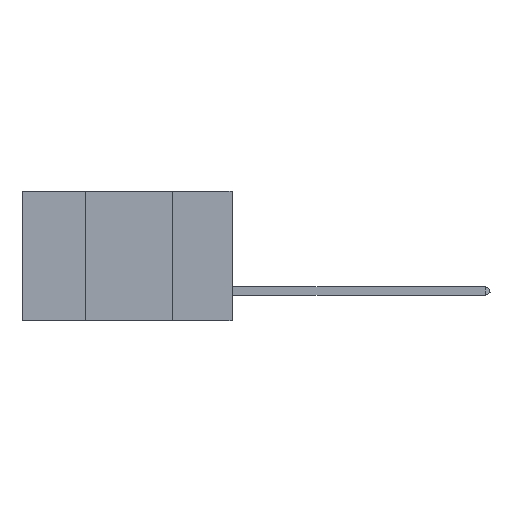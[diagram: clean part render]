
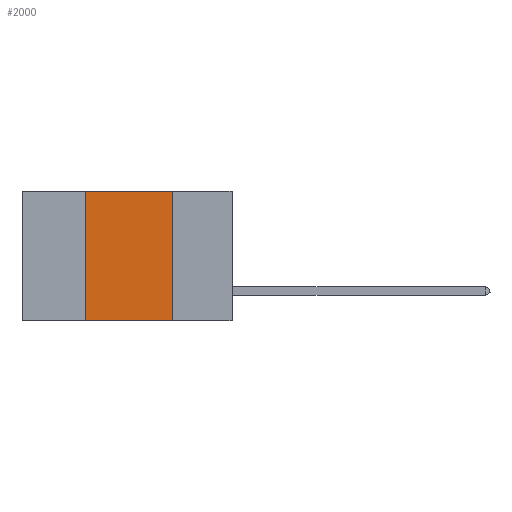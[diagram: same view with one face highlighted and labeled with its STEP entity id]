
A CAD part, left-side view. The second image highlights one B-rep face of the part: STEP entity #2000.
In plain terms, the highlighted planar face has unit normal (-1, 0, 0).
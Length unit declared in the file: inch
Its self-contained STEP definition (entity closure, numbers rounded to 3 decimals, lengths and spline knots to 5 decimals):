
#184 = PLANE ( 'NONE',  #1327 ) ;
#1327 = AXIS2_PLACEMENT_3D ( 'NONE', #18711, #16907, #7871 ) ;
#1763 = VERTEX_POINT ( 'NONE', #6964 ) ;
#2000 = ADVANCED_FACE ( 'NONE', ( #18683 ), #184, .F. ) ;
#2273 = VECTOR ( 'NONE', #9489, 39.37008 ) ;
#4126 = EDGE_CURVE ( 'NONE', #18324, #16818, #17830, .T. ) ;
#4892 = CARTESIAN_POINT ( 'NONE',  ( 0., 0.6, -0.37 ) ) ;
#5587 = CARTESIAN_POINT ( 'NONE',  ( 0., 0.17, 0. ) ) ;
#5829 = CARTESIAN_POINT ( 'NONE',  ( 0., 0.17, 0. ) ) ;
#6475 = EDGE_LOOP ( 'NONE', ( #11218, #17809, #11606, #12803 ) ) ;
#6964 = CARTESIAN_POINT ( 'NONE',  ( 0., 0.42, -0.37 ) ) ;
#7453 = DIRECTION ( 'NONE',  ( 0., 0., -1. ) ) ;
#7871 = DIRECTION ( 'NONE',  ( 0., 0., -1. ) ) ;
#9065 = VERTEX_POINT ( 'NONE', #12505 ) ;
#9489 = DIRECTION ( 'NONE',  ( 0., 0., 1. ) ) ;
#10135 = VECTOR ( 'NONE', #13042, 39.37008 ) ;
#10976 = CARTESIAN_POINT ( 'NONE',  ( 0., 0.42, 0. ) ) ;
#11218 = ORIENTED_EDGE ( 'NONE', *, *, #17366, .F. ) ;
#11259 = DIRECTION ( 'NONE',  ( 0., -1., 0. ) ) ;
#11606 = ORIENTED_EDGE ( 'NONE', *, *, #16121, .F. ) ;
#11933 = EDGE_CURVE ( 'NONE', #1763, #9065, #19930, .T. ) ;
#12505 = CARTESIAN_POINT ( 'NONE',  ( 0., 0.17, -0.37 ) ) ;
#12803 = ORIENTED_EDGE ( 'NONE', *, *, #11933, .T. ) ;
#12872 = VECTOR ( 'NONE', #11259, 39.37008 ) ;
#13042 = DIRECTION ( 'NONE',  ( 0., -1., 0. ) ) ;
#13316 = VECTOR ( 'NONE', #7453, 39.37008 ) ;
#15065 = LINE ( 'NONE', #10976, #2273 ) ;
#16121 = EDGE_CURVE ( 'NONE', #1763, #18324, #15065, .T. ) ;
#16141 = CARTESIAN_POINT ( 'NONE',  ( 0., 0.42, 0. ) ) ;
#16818 = VERTEX_POINT ( 'NONE', #5587 ) ;
#16907 = DIRECTION ( 'NONE',  ( 1., 0., 0. ) ) ;
#17366 = EDGE_CURVE ( 'NONE', #16818, #9065, #18175, .T. ) ;
#17809 = ORIENTED_EDGE ( 'NONE', *, *, #4126, .F. ) ;
#17830 = LINE ( 'NONE', #19220, #10135 ) ;
#18175 = LINE ( 'NONE', #5829, #13316 ) ;
#18324 = VERTEX_POINT ( 'NONE', #16141 ) ;
#18683 = FACE_OUTER_BOUND ( 'NONE', #6475, .T. ) ;
#18711 = CARTESIAN_POINT ( 'NONE',  ( 0., 0.6, 0. ) ) ;
#19220 = CARTESIAN_POINT ( 'NONE',  ( 0., 0.6, 0. ) ) ;
#19930 = LINE ( 'NONE', #4892, #12872 ) ;
